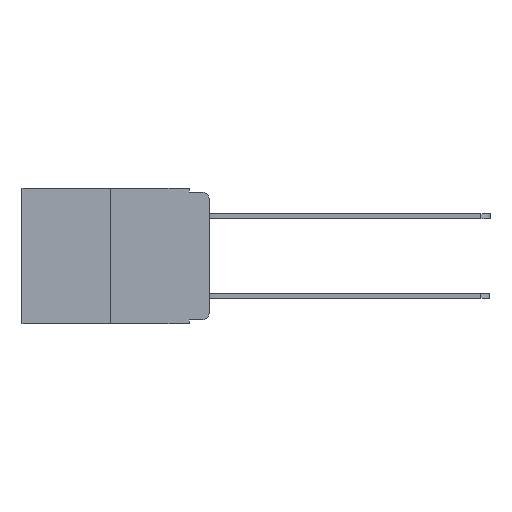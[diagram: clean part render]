
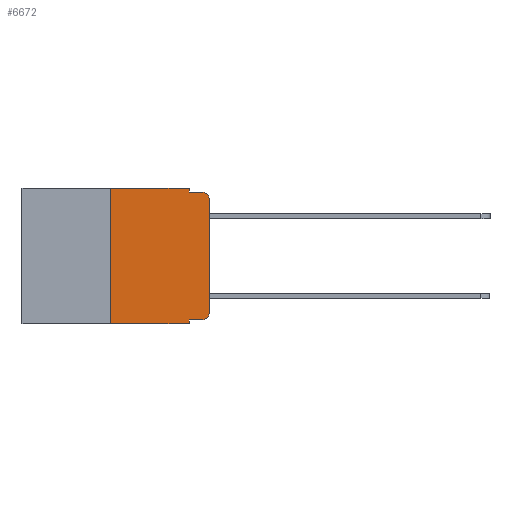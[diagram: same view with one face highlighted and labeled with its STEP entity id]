
A CAD part, left-side view. The second image highlights one B-rep face of the part: STEP entity #6672.
In plain terms, the highlighted planar face has unit normal (-1, 0, 0).
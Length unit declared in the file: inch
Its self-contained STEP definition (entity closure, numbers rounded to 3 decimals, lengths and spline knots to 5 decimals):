
#22 = ORIENTED_EDGE ( 'NONE', *, *, #10778, .F. ) ;
#30 = AXIS2_PLACEMENT_3D ( 'NONE', #12823, #4554, #16082 ) ;
#222 = ORIENTED_EDGE ( 'NONE', *, *, #1551, .T. ) ;
#242 = CARTESIAN_POINT ( 'NONE',  ( 0., 0.25, 0. ) ) ;
#245 = ORIENTED_EDGE ( 'NONE', *, *, #5392, .T. ) ;
#697 = VERTEX_POINT ( 'NONE', #4864 ) ;
#873 = VECTOR ( 'NONE', #18276, 39.37008 ) ;
#1096 = DIRECTION ( 'NONE',  ( -1., 0., 0. ) ) ;
#1551 = EDGE_CURVE ( 'NONE', #17878, #16563, #18490, .T. ) ;
#1566 = CARTESIAN_POINT ( 'NONE',  ( 0., 0.051, 0. ) ) ;
#1710 = FACE_OUTER_BOUND ( 'NONE', #8774, .T. ) ;
#1934 = VERTEX_POINT ( 'NONE', #18307 ) ;
#2358 = ORIENTED_EDGE ( 'NONE', *, *, #17208, .F. ) ;
#2638 = ORIENTED_EDGE ( 'NONE', *, *, #8292, .T. ) ;
#2653 = AXIS2_PLACEMENT_3D ( 'NONE', #11269, #1096, #12904 ) ;
#2877 = ORIENTED_EDGE ( 'NONE', *, *, #7360, .F. ) ;
#3149 = EDGE_CURVE ( 'NONE', #20007, #17878, #15958, .T. ) ;
#3843 = DIRECTION ( 'NONE',  ( 0., 0., 1. ) ) ;
#4318 = ORIENTED_EDGE ( 'NONE', *, *, #18939, .T. ) ;
#4525 = DIRECTION ( 'NONE',  ( 0., -1., 0. ) ) ;
#4554 = DIRECTION ( 'NONE',  ( 1., 0., 0. ) ) ;
#4864 = CARTESIAN_POINT ( 'NONE',  ( 0., 0.02, -0.01 ) ) ;
#5273 = VECTOR ( 'NONE', #20680, 39.37008 ) ;
#5304 = LINE ( 'NONE', #15384, #13185 ) ;
#5359 = CARTESIAN_POINT ( 'NONE',  ( 0., 0., -0.03 ) ) ;
#5392 = EDGE_CURVE ( 'NONE', #16563, #697, #20893, .T. ) ;
#5566 = CARTESIAN_POINT ( 'NONE',  ( 0., 0.02, -0.03 ) ) ;
#5757 = VECTOR ( 'NONE', #15821, 39.37008 ) ;
#6041 = CARTESIAN_POINT ( 'NONE',  ( 0., 0., -0.313 ) ) ;
#6189 = VERTEX_POINT ( 'NONE', #1566 ) ;
#6251 = CARTESIAN_POINT ( 'NONE',  ( 0., 0.051, -0.01 ) ) ;
#6365 = VERTEX_POINT ( 'NONE', #12128 ) ;
#6426 = LINE ( 'NONE', #6251, #19433 ) ;
#6672 = ADVANCED_FACE ( 'NONE', ( #1710 ), #20690, .F. ) ;
#6926 = EDGE_CURVE ( 'NONE', #7439, #15390, #18459, .T. ) ;
#7243 = DIRECTION ( 'NONE',  ( 0., 0., -1. ) ) ;
#7340 = VERTEX_POINT ( 'NONE', #16057 ) ;
#7360 = EDGE_CURVE ( 'NONE', #7340, #697, #6426, .T. ) ;
#7439 = VERTEX_POINT ( 'NONE', #13159 ) ;
#8292 = EDGE_CURVE ( 'NONE', #7439, #6365, #11198, .T. ) ;
#8580 = CARTESIAN_POINT ( 'NONE',  ( 0., 0.25, 0. ) ) ;
#8737 = AXIS2_PLACEMENT_3D ( 'NONE', #5566, #17040, #7243 ) ;
#8774 = EDGE_LOOP ( 'NONE', ( #222, #245, #2877, #22, #2358, #20636, #2638, #13906, #4318, #10791 ) ) ;
#8792 = CARTESIAN_POINT ( 'NONE',  ( 0., 0.02, -0.333 ) ) ;
#10678 = VECTOR ( 'NONE', #10681, 39.37008 ) ;
#10681 = DIRECTION ( 'NONE',  ( 0., -1., 0. ) ) ;
#10778 = EDGE_CURVE ( 'NONE', #6189, #7340, #19791, .T. ) ;
#10791 = ORIENTED_EDGE ( 'NONE', *, *, #3149, .T. ) ;
#11198 = LINE ( 'NONE', #18642, #10678 ) ;
#11269 = CARTESIAN_POINT ( 'NONE',  ( 0., 0.02, -0.313 ) ) ;
#11669 = LINE ( 'NONE', #14634, #19607 ) ;
#12128 = CARTESIAN_POINT ( 'NONE',  ( 0., 0.051, -0.343 ) ) ;
#12823 = CARTESIAN_POINT ( 'NONE',  ( 0., 0.473, 0. ) ) ;
#12904 = DIRECTION ( 'NONE',  ( 0., 0., -1. ) ) ;
#12945 = CARTESIAN_POINT ( 'NONE',  ( 0., 0., 0. ) ) ;
#13159 = CARTESIAN_POINT ( 'NONE',  ( 0., 0.25, -0.343 ) ) ;
#13185 = VECTOR ( 'NONE', #16960, 39.37008 ) ;
#13628 = LINE ( 'NONE', #14251, #5757 ) ;
#13906 = ORIENTED_EDGE ( 'NONE', *, *, #15767, .F. ) ;
#14251 = CARTESIAN_POINT ( 'NONE',  ( 0., 0.051, -0.333 ) ) ;
#14634 = CARTESIAN_POINT ( 'NONE',  ( 0., 0.051, 0. ) ) ;
#15384 = CARTESIAN_POINT ( 'NONE',  ( 0., 0.473, 0. ) ) ;
#15390 = VERTEX_POINT ( 'NONE', #242 ) ;
#15767 = EDGE_CURVE ( 'NONE', #1934, #6365, #11669, .T. ) ;
#15821 = DIRECTION ( 'NONE',  ( 0., -1., 0. ) ) ;
#15958 = CIRCLE ( 'NONE', #2653, 0.02 ) ;
#16057 = CARTESIAN_POINT ( 'NONE',  ( 0., 0.051, -0.01 ) ) ;
#16082 = DIRECTION ( 'NONE',  ( 0., 0., -1. ) ) ;
#16205 = DIRECTION ( 'NONE',  ( 0., 0., -1. ) ) ;
#16563 = VERTEX_POINT ( 'NONE', #5359 ) ;
#16960 = DIRECTION ( 'NONE',  ( 0., -1., 0. ) ) ;
#17040 = DIRECTION ( 'NONE',  ( -1., 0., 0. ) ) ;
#17208 = EDGE_CURVE ( 'NONE', #15390, #6189, #5304, .T. ) ;
#17646 = CARTESIAN_POINT ( 'NONE',  ( 0., 0.051, 0. ) ) ;
#17878 = VERTEX_POINT ( 'NONE', #6041 ) ;
#17978 = VECTOR ( 'NONE', #3843, 39.37008 ) ;
#18276 = DIRECTION ( 'NONE',  ( 0., 0., 1. ) ) ;
#18307 = CARTESIAN_POINT ( 'NONE',  ( 0., 0.051, -0.333 ) ) ;
#18459 = LINE ( 'NONE', #8580, #873 ) ;
#18490 = LINE ( 'NONE', #12945, #17978 ) ;
#18642 = CARTESIAN_POINT ( 'NONE',  ( 0., 0.473, -0.343 ) ) ;
#18939 = EDGE_CURVE ( 'NONE', #1934, #20007, #13628, .T. ) ;
#19433 = VECTOR ( 'NONE', #4525, 39.37008 ) ;
#19607 = VECTOR ( 'NONE', #16205, 39.37008 ) ;
#19791 = LINE ( 'NONE', #17646, #5273 ) ;
#20007 = VERTEX_POINT ( 'NONE', #8792 ) ;
#20636 = ORIENTED_EDGE ( 'NONE', *, *, #6926, .F. ) ;
#20680 = DIRECTION ( 'NONE',  ( 0., 0., -1. ) ) ;
#20690 = PLANE ( 'NONE',  #30 ) ;
#20893 = CIRCLE ( 'NONE', #8737, 0.02 ) ;
